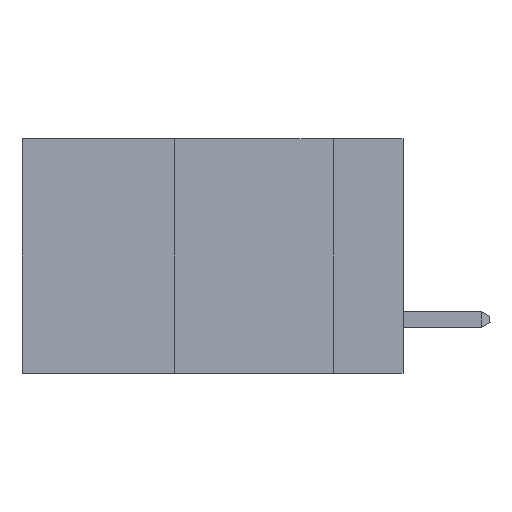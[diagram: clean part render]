
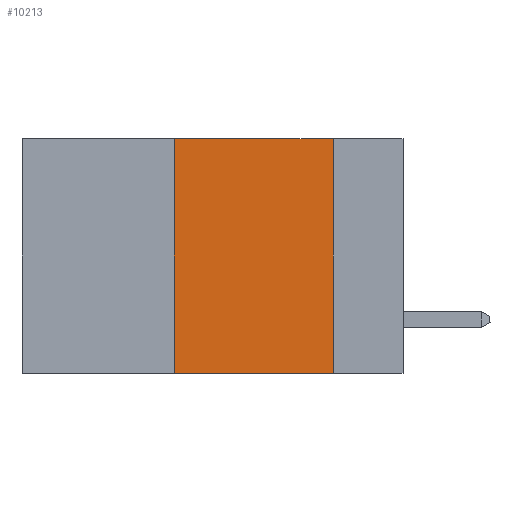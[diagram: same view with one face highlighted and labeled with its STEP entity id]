
A CAD part, left-side view. The second image highlights one B-rep face of the part: STEP entity #10213.
In plain terms, the highlighted planar face has unit normal (-1, 0, 0).
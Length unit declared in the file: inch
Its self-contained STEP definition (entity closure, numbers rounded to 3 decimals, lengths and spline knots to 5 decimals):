
#37 = DIRECTION ( 'NONE',  ( 0., 0., 1. ) ) ;
#1206 = CARTESIAN_POINT ( 'NONE',  ( 0., 0.6, 0. ) ) ;
#1350 = CARTESIAN_POINT ( 'NONE',  ( 0., 0.6, 0. ) ) ;
#2299 = VERTEX_POINT ( 'NONE', #8865 ) ;
#2939 = CARTESIAN_POINT ( 'NONE',  ( 0., 0.36, -0.37 ) ) ;
#3177 = DIRECTION ( 'NONE',  ( 0., 0., -1. ) ) ;
#3317 = DIRECTION ( 'NONE',  ( 0., -1., 0. ) ) ;
#3426 = PLANE ( 'NONE',  #16812 ) ;
#4131 = ORIENTED_EDGE ( 'NONE', *, *, #8053, .F. ) ;
#4247 = DIRECTION ( 'NONE',  ( 0., 0., -1. ) ) ;
#5315 = ORIENTED_EDGE ( 'NONE', *, *, #7248, .F. ) ;
#5876 = VECTOR ( 'NONE', #37, 39.37008 ) ;
#6400 = VERTEX_POINT ( 'NONE', #20303 ) ;
#7248 = EDGE_CURVE ( 'NONE', #6400, #22829, #24878, .T. ) ;
#7302 = DIRECTION ( 'NONE',  ( 1., 0., 0. ) ) ;
#7919 = CARTESIAN_POINT ( 'NONE',  ( 0., 0.11, 0. ) ) ;
#8053 = EDGE_CURVE ( 'NONE', #20586, #6400, #23045, .T. ) ;
#8234 = EDGE_CURVE ( 'NONE', #22829, #2299, #8583, .T. ) ;
#8583 = LINE ( 'NONE', #10971, #18233 ) ;
#8620 = ORIENTED_EDGE ( 'NONE', *, *, #8234, .F. ) ;
#8865 = CARTESIAN_POINT ( 'NONE',  ( 0., 0.11, -0.37 ) ) ;
#8949 = LINE ( 'NONE', #10294, #9246 ) ;
#9246 = VECTOR ( 'NONE', #11635, 39.37008 ) ;
#9769 = ORIENTED_EDGE ( 'NONE', *, *, #16754, .T. ) ;
#10213 = ADVANCED_FACE ( 'NONE', ( #10232 ), #3426, .F. ) ;
#10232 = FACE_OUTER_BOUND ( 'NONE', #13671, .T. ) ;
#10294 = CARTESIAN_POINT ( 'NONE',  ( 0., 0.6, -0.37 ) ) ;
#10783 = VECTOR ( 'NONE', #3317, 39.37008 ) ;
#10971 = CARTESIAN_POINT ( 'NONE',  ( 0., 0.11, 0. ) ) ;
#11635 = DIRECTION ( 'NONE',  ( 0., -1., 0. ) ) ;
#13671 = EDGE_LOOP ( 'NONE', ( #8620, #5315, #4131, #9769 ) ) ;
#16754 = EDGE_CURVE ( 'NONE', #20586, #2299, #8949, .T. ) ;
#16812 = AXIS2_PLACEMENT_3D ( 'NONE', #1206, #7302, #3177 ) ;
#18233 = VECTOR ( 'NONE', #4247, 39.37008 ) ;
#20303 = CARTESIAN_POINT ( 'NONE',  ( 0., 0.36, 0. ) ) ;
#20586 = VERTEX_POINT ( 'NONE', #2939 ) ;
#21178 = CARTESIAN_POINT ( 'NONE',  ( 0., 0.36, 0. ) ) ;
#22829 = VERTEX_POINT ( 'NONE', #7919 ) ;
#23045 = LINE ( 'NONE', #21178, #5876 ) ;
#24878 = LINE ( 'NONE', #1350, #10783 ) ;
